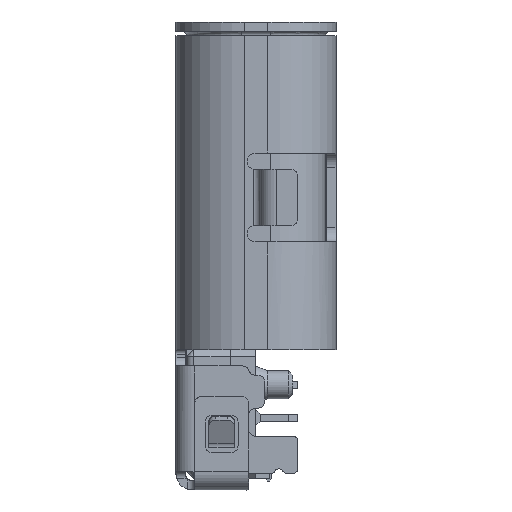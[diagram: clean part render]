
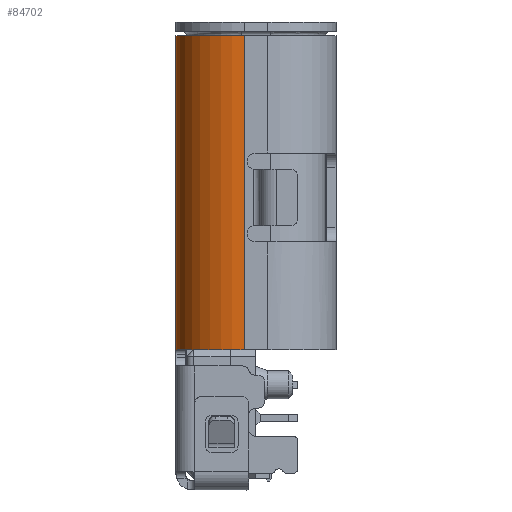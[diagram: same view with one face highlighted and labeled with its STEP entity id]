
A CAD part, left-side view. The second image highlights one B-rep face of the part: STEP entity #84702.
In plain terms, the highlighted cylindrical face has radius 1.46 mm (diameter 2.92 mm), a partial arc.
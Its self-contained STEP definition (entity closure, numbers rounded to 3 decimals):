
#785 = ORIENTED_EDGE ( 'NONE', *, *, #90117, .T. ) ;
#6807 = EDGE_CURVE ( 'NONE', #73547, #115519, #34045, .T. ) ;
#10803 = DIRECTION ( 'NONE',  ( 1., 0., 0. ) ) ;
#16011 = LINE ( 'NONE', #41235, #62484 ) ;
#19506 = CARTESIAN_POINT ( 'NONE',  ( -81.312, 8.889, -12.651 ) ) ;
#19645 = CIRCLE ( 'NONE', #107795, 1.46 ) ;
#28439 = AXIS2_PLACEMENT_3D ( 'NONE', #112610, #32039, #67873 ) ;
#32039 = DIRECTION ( 'NONE',  ( 0., 0., -1. ) ) ;
#34045 = CIRCLE ( 'NONE', #28439, 1.46 ) ;
#38705 = EDGE_CURVE ( 'NONE', #115519, #66683, #16011, .T. ) ;
#40822 = CARTESIAN_POINT ( 'NONE',  ( -82.772, 7.429, -19.361 ) ) ;
#41235 = CARTESIAN_POINT ( 'NONE',  ( -82.772, 7.429, -17.331 ) ) ;
#44516 = FACE_OUTER_BOUND ( 'NONE', #106484, .T. ) ;
#47399 = VERTEX_POINT ( 'NONE', #86434 ) ;
#52184 = DIRECTION ( 'NONE',  ( 0., 0., 1. ) ) ;
#60615 = DIRECTION ( 'NONE',  ( 0., 0., -1. ) ) ;
#60734 = ORIENTED_EDGE ( 'NONE', *, *, #63939, .T. ) ;
#61463 = ORIENTED_EDGE ( 'NONE', *, *, #6807, .T. ) ;
#62484 = VECTOR ( 'NONE', #60615, 1000. ) ;
#63939 = EDGE_CURVE ( 'NONE', #66683, #47399, #19645, .T. ) ;
#66358 = LINE ( 'NONE', #103341, #75045 ) ;
#66683 = VERTEX_POINT ( 'NONE', #40822 ) ;
#67873 = DIRECTION ( 'NONE',  ( 1., 0., 0. ) ) ;
#70383 = DIRECTION ( 'NONE',  ( 1., 0., 0. ) ) ;
#73033 = CARTESIAN_POINT ( 'NONE',  ( -82.772, 8.889, -19.361 ) ) ;
#73547 = VERTEX_POINT ( 'NONE', #19506 ) ;
#75045 = VECTOR ( 'NONE', #112228, 1000. ) ;
#80335 = CARTESIAN_POINT ( 'NONE',  ( -82.772, 8.889, -19.495 ) ) ;
#84702 = ADVANCED_FACE ( 'NONE', ( #44516 ), #88620, .T. ) ;
#86434 = CARTESIAN_POINT ( 'NONE',  ( -81.312, 8.889, -19.361 ) ) ;
#88620 = CYLINDRICAL_SURFACE ( 'NONE', #104243, 1.46 ) ;
#90117 = EDGE_CURVE ( 'NONE', #47399, #73547, #66358, .T. ) ;
#99760 = ORIENTED_EDGE ( 'NONE', *, *, #38705, .T. ) ;
#103341 = CARTESIAN_POINT ( 'NONE',  ( -81.312, 8.889, -19.495 ) ) ;
#104243 = AXIS2_PLACEMENT_3D ( 'NONE', #80335, #52184, #70383 ) ;
#106484 = EDGE_LOOP ( 'NONE', ( #99760, #60734, #785, #61463 ) ) ;
#107795 = AXIS2_PLACEMENT_3D ( 'NONE', #73033, #108919, #10803 ) ;
#108919 = DIRECTION ( 'NONE',  ( 0., 0., 1. ) ) ;
#112228 = DIRECTION ( 'NONE',  ( 0., 0., 1. ) ) ;
#112394 = CARTESIAN_POINT ( 'NONE',  ( -82.772, 7.429, -12.651 ) ) ;
#112610 = CARTESIAN_POINT ( 'NONE',  ( -82.772, 8.889, -12.651 ) ) ;
#115519 = VERTEX_POINT ( 'NONE', #112394 ) ;
